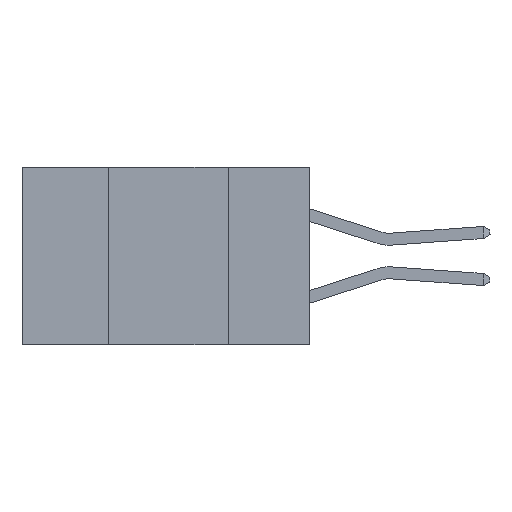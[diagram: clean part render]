
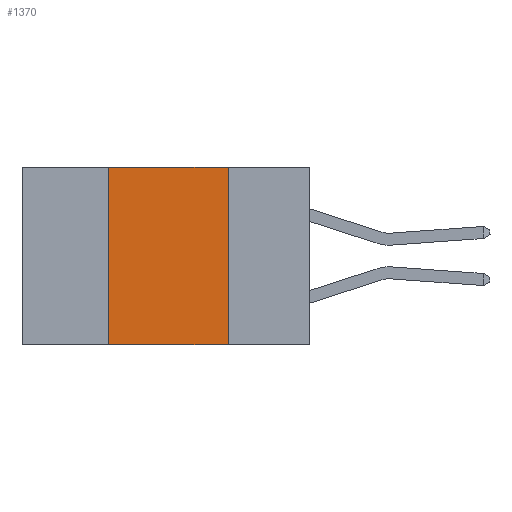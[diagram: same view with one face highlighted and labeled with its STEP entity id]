
A CAD part, left-side view. The second image highlights one B-rep face of the part: STEP entity #1370.
In plain terms, the highlighted planar face has unit normal (-1, 0, 0).
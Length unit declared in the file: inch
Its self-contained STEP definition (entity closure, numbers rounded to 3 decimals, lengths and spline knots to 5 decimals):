
#681 = CARTESIAN_POINT ( 'NONE',  ( 0., 0.17, -0.37 ) ) ;
#692 = VECTOR ( 'NONE', #7682, 39.37008 ) ;
#1251 = LINE ( 'NONE', #7866, #4905 ) ;
#1370 = ADVANCED_FACE ( 'NONE', ( #2609 ), #1541, .F. ) ;
#1541 = PLANE ( 'NONE',  #6169 ) ;
#1570 = DIRECTION ( 'NONE',  ( 1., 0., 0. ) ) ;
#1714 = CARTESIAN_POINT ( 'NONE',  ( 0., 0.6, 0. ) ) ;
#2118 = EDGE_CURVE ( 'NONE', #3186, #7729, #8097, .T. ) ;
#2119 = EDGE_CURVE ( 'NONE', #3260, #3186, #5087, .T. ) ;
#2131 = EDGE_CURVE ( 'NONE', #4503, #3260, #1251, .T. ) ;
#2134 = EDGE_CURVE ( 'NONE', #4503, #7729, #6460, .T. ) ;
#2335 = DIRECTION ( 'NONE',  ( 0., 0., -1. ) ) ;
#2609 = FACE_OUTER_BOUND ( 'NONE', #5008, .T. ) ;
#3186 = VERTEX_POINT ( 'NONE', #6012 ) ;
#3226 = VECTOR ( 'NONE', #7956, 39.37008 ) ;
#3260 = VERTEX_POINT ( 'NONE', #6768 ) ;
#3909 = ORIENTED_EDGE ( 'NONE', *, *, #2119, .F. ) ;
#4503 = VERTEX_POINT ( 'NONE', #5766 ) ;
#4905 = VECTOR ( 'NONE', #7959, 39.37008 ) ;
#5008 = EDGE_LOOP ( 'NONE', ( #8441, #3909, #5639, #7141 ) ) ;
#5087 = LINE ( 'NONE', #7874, #7936 ) ;
#5639 = ORIENTED_EDGE ( 'NONE', *, *, #2131, .F. ) ;
#5766 = CARTESIAN_POINT ( 'NONE',  ( 0., 0.42, -0.37 ) ) ;
#6012 = CARTESIAN_POINT ( 'NONE',  ( 0., 0.17, 0. ) ) ;
#6169 = AXIS2_PLACEMENT_3D ( 'NONE', #1714, #1570, #2335 ) ;
#6460 = LINE ( 'NONE', #7786, #692 ) ;
#6768 = CARTESIAN_POINT ( 'NONE',  ( 0., 0.42, 0. ) ) ;
#7141 = ORIENTED_EDGE ( 'NONE', *, *, #2134, .T. ) ;
#7682 = DIRECTION ( 'NONE',  ( 0., -1., 0. ) ) ;
#7729 = VERTEX_POINT ( 'NONE', #681 ) ;
#7786 = CARTESIAN_POINT ( 'NONE',  ( 0., 0.6, -0.37 ) ) ;
#7807 = DIRECTION ( 'NONE',  ( 0., -1., 0. ) ) ;
#7866 = CARTESIAN_POINT ( 'NONE',  ( 0., 0.42, -0.37 ) ) ;
#7874 = CARTESIAN_POINT ( 'NONE',  ( 0., 0.6, 0. ) ) ;
#7936 = VECTOR ( 'NONE', #7807, 39.37008 ) ;
#7956 = DIRECTION ( 'NONE',  ( 0., 0., -1. ) ) ;
#7959 = DIRECTION ( 'NONE',  ( 0., 0., 1. ) ) ;
#8097 = LINE ( 'NONE', #8161, #3226 ) ;
#8161 = CARTESIAN_POINT ( 'NONE',  ( 0., 0.17, -0.37 ) ) ;
#8441 = ORIENTED_EDGE ( 'NONE', *, *, #2118, .F. ) ;
